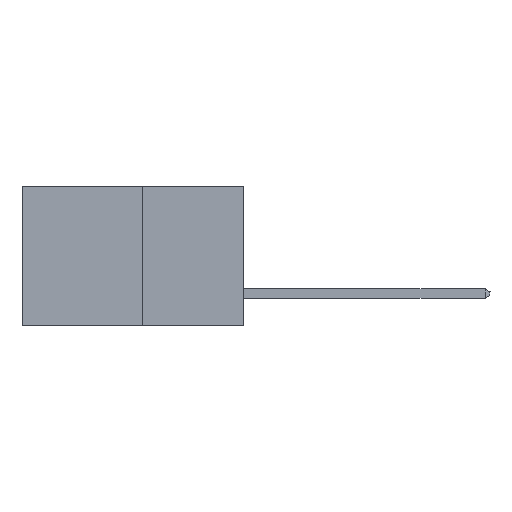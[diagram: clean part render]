
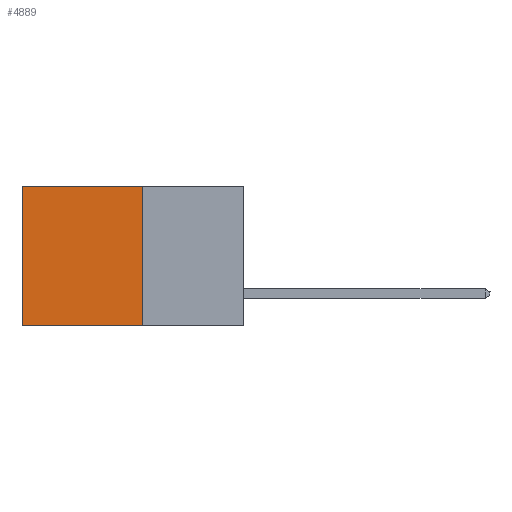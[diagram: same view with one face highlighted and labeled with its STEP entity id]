
A CAD part, left-side view. The second image highlights one B-rep face of the part: STEP entity #4889.
In plain terms, the highlighted planar face has unit normal (-1, 0, 0).
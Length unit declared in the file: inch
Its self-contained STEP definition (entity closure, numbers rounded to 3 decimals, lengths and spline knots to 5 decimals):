
#99 = ORIENTED_EDGE ( 'NONE', *, *, #2097, .T. ) ;
#896 = CARTESIAN_POINT ( 'NONE',  ( 0.277, 0.27, -0.37 ) ) ;
#1485 = EDGE_CURVE ( 'NONE', #13374, #3311, #7884, .T. ) ;
#1686 = DIRECTION ( 'NONE',  ( 0., 1., 0. ) ) ;
#2097 = EDGE_CURVE ( 'NONE', #5378, #5575, #8742, .T. ) ;
#2668 = DIRECTION ( 'NONE',  ( 0., 0., -1. ) ) ;
#3247 = CARTESIAN_POINT ( 'NONE',  ( 0.277, 0.27, 0. ) ) ;
#3311 = VERTEX_POINT ( 'NONE', #10353 ) ;
#3891 = ORIENTED_EDGE ( 'NONE', *, *, #10545, .T. ) ;
#4017 = CARTESIAN_POINT ( 'NONE',  ( 0.277, 0.27, -0.37 ) ) ;
#4066 = DIRECTION ( 'NONE',  ( 0., 0., -1. ) ) ;
#4395 = EDGE_CURVE ( 'NONE', #3311, #5575, #12116, .T. ) ;
#4889 = ADVANCED_FACE ( 'NONE', ( #13602 ), #11911, .F. ) ;
#5006 = EDGE_LOOP ( 'NONE', ( #99, #7941, #13783, #3891 ) ) ;
#5330 = AXIS2_PLACEMENT_3D ( 'NONE', #13214, #13209, #13288 ) ;
#5378 = VERTEX_POINT ( 'NONE', #10378 ) ;
#5575 = VERTEX_POINT ( 'NONE', #7602 ) ;
#5735 = VECTOR ( 'NONE', #2668, 39.37008 ) ;
#7602 = CARTESIAN_POINT ( 'NONE',  ( 0.277, 0.59, -0.37 ) ) ;
#7884 = LINE ( 'NONE', #4017, #13361 ) ;
#7941 = ORIENTED_EDGE ( 'NONE', *, *, #4395, .F. ) ;
#8497 = VECTOR ( 'NONE', #1686, 39.37008 ) ;
#8742 = LINE ( 'NONE', #9343, #5735 ) ;
#9325 = VECTOR ( 'NONE', #10684, 39.37008 ) ;
#9343 = CARTESIAN_POINT ( 'NONE',  ( 0.277, 0.59, -0.37 ) ) ;
#10353 = CARTESIAN_POINT ( 'NONE',  ( 0.277, 0.27, -0.37 ) ) ;
#10378 = CARTESIAN_POINT ( 'NONE',  ( 0.277, 0.59, 0. ) ) ;
#10545 = EDGE_CURVE ( 'NONE', #13374, #5378, #11902, .T. ) ;
#10684 = DIRECTION ( 'NONE',  ( 0., 1., 0. ) ) ;
#10700 = CARTESIAN_POINT ( 'NONE',  ( 0.277, 0.27, 0. ) ) ;
#11902 = LINE ( 'NONE', #10700, #9325 ) ;
#11911 = PLANE ( 'NONE',  #5330 ) ;
#12116 = LINE ( 'NONE', #896, #8497 ) ;
#13209 = DIRECTION ( 'NONE',  ( 1., 0., 0. ) ) ;
#13214 = CARTESIAN_POINT ( 'NONE',  ( 0.277, 0.27, -0.37 ) ) ;
#13288 = DIRECTION ( 'NONE',  ( 0., 0., -1. ) ) ;
#13361 = VECTOR ( 'NONE', #4066, 39.37008 ) ;
#13374 = VERTEX_POINT ( 'NONE', #3247 ) ;
#13602 = FACE_OUTER_BOUND ( 'NONE', #5006, .T. ) ;
#13783 = ORIENTED_EDGE ( 'NONE', *, *, #1485, .F. ) ;
